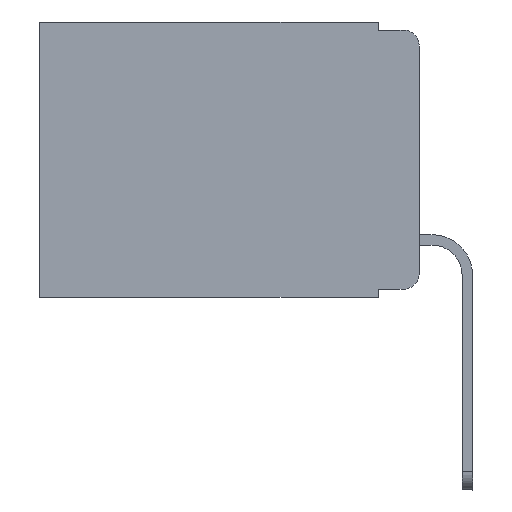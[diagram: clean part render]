
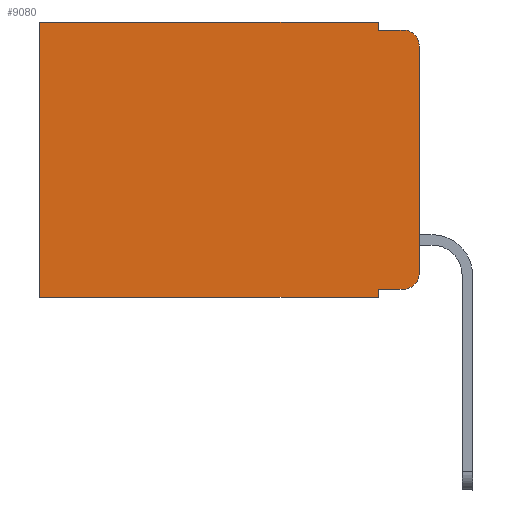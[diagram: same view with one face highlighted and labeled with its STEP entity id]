
A CAD part, left-side view. The second image highlights one B-rep face of the part: STEP entity #9080.
In plain terms, the highlighted planar face has unit normal (-1, 0, 0).
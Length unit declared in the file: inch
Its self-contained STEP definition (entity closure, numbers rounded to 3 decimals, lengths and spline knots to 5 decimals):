
#231 = DIRECTION ( 'NONE',  ( -1., 0., 0. ) ) ;
#303 = EDGE_LOOP ( 'NONE', ( #11799, #6072, #9028, #1804, #1176, #7500, #7277, #16498, #19898, #20411 ) ) ;
#416 = CARTESIAN_POINT ( 'NONE',  ( 0.298, 0., -0.03 ) ) ;
#450 = CARTESIAN_POINT ( 'NONE',  ( 0.298, 0.051, -0.01 ) ) ;
#621 = PLANE ( 'NONE',  #7052 ) ;
#1028 = DIRECTION ( 'NONE',  ( 0., 1., 0. ) ) ;
#1176 = ORIENTED_EDGE ( 'NONE', *, *, #7925, .T. ) ;
#1417 = EDGE_CURVE ( 'NONE', #14466, #8694, #9515, .T. ) ;
#1769 = DIRECTION ( 'NONE',  ( 0., 0., -1. ) ) ;
#1804 = ORIENTED_EDGE ( 'NONE', *, *, #1417, .F. ) ;
#2060 = VERTEX_POINT ( 'NONE', #5560 ) ;
#2074 = CARTESIAN_POINT ( 'NONE',  ( 0.298, 0.473, 0. ) ) ;
#2204 = CARTESIAN_POINT ( 'NONE',  ( 0.298, 0.473, -0.343 ) ) ;
#2429 = VERTEX_POINT ( 'NONE', #16577 ) ;
#3120 = DIRECTION ( 'NONE',  ( 0., 0., -1. ) ) ;
#3481 = EDGE_CURVE ( 'NONE', #8694, #13487, #6338, .T. ) ;
#3748 = CARTESIAN_POINT ( 'NONE',  ( 0.298, 0., -0.313 ) ) ;
#4285 = EDGE_CURVE ( 'NONE', #2060, #18305, #8855, .T. ) ;
#4307 = CARTESIAN_POINT ( 'NONE',  ( 0.298, 0., 0. ) ) ;
#4752 = CARTESIAN_POINT ( 'NONE',  ( 0.298, 0.051, 0. ) ) ;
#5083 = DIRECTION ( 'NONE',  ( 0., -1., 0. ) ) ;
#5377 = VERTEX_POINT ( 'NONE', #416 ) ;
#5560 = CARTESIAN_POINT ( 'NONE',  ( 0.298, 0.051, -0.343 ) ) ;
#6072 = ORIENTED_EDGE ( 'NONE', *, *, #19888, .T. ) ;
#6338 = LINE ( 'NONE', #12645, #11651 ) ;
#6442 = CARTESIAN_POINT ( 'NONE',  ( 0.298, 0.473, 0. ) ) ;
#6527 = CARTESIAN_POINT ( 'NONE',  ( 0.298, 0.02, -0.313 ) ) ;
#6745 = EDGE_CURVE ( 'NONE', #12764, #11476, #6968, .T. ) ;
#6900 = DIRECTION ( 'NONE',  ( -1., 0., 0. ) ) ;
#6968 = CIRCLE ( 'NONE', #15557, 0.02 ) ;
#7052 = AXIS2_PLACEMENT_3D ( 'NONE', #13111, #19425, #11381 ) ;
#7158 = VECTOR ( 'NONE', #16345, 39.37008 ) ;
#7217 = VECTOR ( 'NONE', #1769, 39.37008 ) ;
#7277 = ORIENTED_EDGE ( 'NONE', *, *, #4285, .F. ) ;
#7319 = CIRCLE ( 'NONE', #10295, 0.02 ) ;
#7391 = LINE ( 'NONE', #14920, #7158 ) ;
#7467 = CARTESIAN_POINT ( 'NONE',  ( 0.298, 0.02, -0.333 ) ) ;
#7500 = ORIENTED_EDGE ( 'NONE', *, *, #15737, .T. ) ;
#7569 = CARTESIAN_POINT ( 'NONE',  ( 0.298, 0.051, 0. ) ) ;
#7925 = EDGE_CURVE ( 'NONE', #14466, #9689, #20003, .T. ) ;
#7940 = VECTOR ( 'NONE', #20174, 39.37008 ) ;
#8359 = LINE ( 'NONE', #2074, #7217 ) ;
#8360 = VECTOR ( 'NONE', #1028, 39.37008 ) ;
#8481 = DIRECTION ( 'NONE',  ( 0., 0., -1. ) ) ;
#8694 = VERTEX_POINT ( 'NONE', #450 ) ;
#8855 = LINE ( 'NONE', #10749, #8360 ) ;
#9028 = ORIENTED_EDGE ( 'NONE', *, *, #3481, .F. ) ;
#9080 = ADVANCED_FACE ( 'NONE', ( #12808 ), #621, .F. ) ;
#9515 = LINE ( 'NONE', #7569, #7940 ) ;
#9689 = VERTEX_POINT ( 'NONE', #6442 ) ;
#10295 = AXIS2_PLACEMENT_3D ( 'NONE', #14853, #6900, #13000 ) ;
#10749 = CARTESIAN_POINT ( 'NONE',  ( 0.298, 0., -0.343 ) ) ;
#11381 = DIRECTION ( 'NONE',  ( 0., 0., -1. ) ) ;
#11386 = CARTESIAN_POINT ( 'NONE',  ( 0.298, 0.051, -0.333 ) ) ;
#11476 = VERTEX_POINT ( 'NONE', #3748 ) ;
#11651 = VECTOR ( 'NONE', #18940, 39.37008 ) ;
#11799 = ORIENTED_EDGE ( 'NONE', *, *, #15068, .F. ) ;
#12645 = CARTESIAN_POINT ( 'NONE',  ( 0.298, 0.051, -0.01 ) ) ;
#12764 = VERTEX_POINT ( 'NONE', #7467 ) ;
#12808 = FACE_OUTER_BOUND ( 'NONE', #303, .T. ) ;
#13000 = DIRECTION ( 'NONE',  ( 0., 0., -1. ) ) ;
#13111 = CARTESIAN_POINT ( 'NONE',  ( 0.298, 0., 0. ) ) ;
#13193 = VECTOR ( 'NONE', #5083, 39.37008 ) ;
#13487 = VERTEX_POINT ( 'NONE', #14926 ) ;
#13494 = DIRECTION ( 'NONE',  ( 0., 1., 0. ) ) ;
#13953 = LINE ( 'NONE', #20152, #16836 ) ;
#14272 = EDGE_CURVE ( 'NONE', #2429, #12764, #19332, .T. ) ;
#14413 = EDGE_CURVE ( 'NONE', #2429, #2060, #13953, .T. ) ;
#14466 = VERTEX_POINT ( 'NONE', #4752 ) ;
#14513 = VECTOR ( 'NONE', #13494, 39.37008 ) ;
#14853 = CARTESIAN_POINT ( 'NONE',  ( 0.298, 0.02, -0.03 ) ) ;
#14920 = CARTESIAN_POINT ( 'NONE',  ( 0.298, 0., 0. ) ) ;
#14926 = CARTESIAN_POINT ( 'NONE',  ( 0.298, 0.02, -0.01 ) ) ;
#15068 = EDGE_CURVE ( 'NONE', #5377, #11476, #7391, .T. ) ;
#15557 = AXIS2_PLACEMENT_3D ( 'NONE', #6527, #231, #8481 ) ;
#15737 = EDGE_CURVE ( 'NONE', #9689, #18305, #8359, .T. ) ;
#16345 = DIRECTION ( 'NONE',  ( 0., 0., -1. ) ) ;
#16498 = ORIENTED_EDGE ( 'NONE', *, *, #14413, .F. ) ;
#16577 = CARTESIAN_POINT ( 'NONE',  ( 0.298, 0.051, -0.333 ) ) ;
#16836 = VECTOR ( 'NONE', #3120, 39.37008 ) ;
#18305 = VERTEX_POINT ( 'NONE', #2204 ) ;
#18940 = DIRECTION ( 'NONE',  ( 0., -1., 0. ) ) ;
#19332 = LINE ( 'NONE', #11386, #13193 ) ;
#19425 = DIRECTION ( 'NONE',  ( 1., 0., 0. ) ) ;
#19888 = EDGE_CURVE ( 'NONE', #5377, #13487, #7319, .T. ) ;
#19898 = ORIENTED_EDGE ( 'NONE', *, *, #14272, .T. ) ;
#20003 = LINE ( 'NONE', #4307, #14513 ) ;
#20152 = CARTESIAN_POINT ( 'NONE',  ( 0.298, 0.051, 0. ) ) ;
#20174 = DIRECTION ( 'NONE',  ( 0., 0., -1. ) ) ;
#20411 = ORIENTED_EDGE ( 'NONE', *, *, #6745, .T. ) ;
